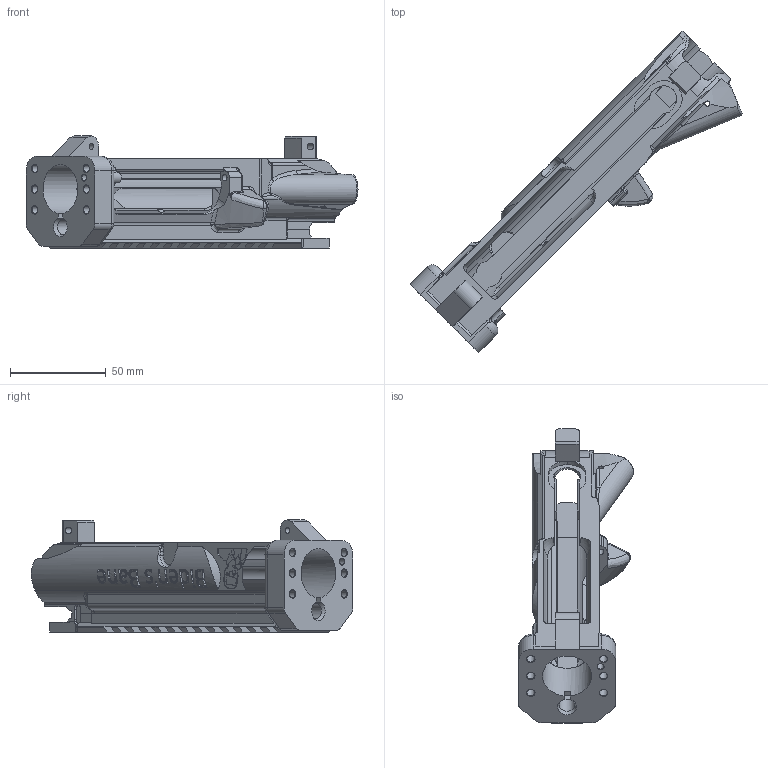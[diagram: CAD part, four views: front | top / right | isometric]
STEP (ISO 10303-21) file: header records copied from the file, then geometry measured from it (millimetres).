
FILE_DESCRIPTION(/* description */ ('STEP AP242','CAx-IF Rec.Pracs.---Representation and Presentation of Product Manufacturing Information (PMI)---4.0---2014-10-13','CAx-IF Rec.Pracs.---3D Tessellated Geometry---0.4---2014-09-14','2;1'),/* implementation_level */ '2;1');
FILE_NAME(/* name */ '62809140d1112b57fbcd074f',/* time_stamp */ '2022-05-15T05:36:02+00:00',/* author */ (''),/* organization */ (''),/* preprocessor_version */ 'ST-DEVELOPER v18.101',/* originating_system */ ' ',/* authorisation */ ' ');
FILE_SCHEMA (('AP242_MANAGED_MODEL_BASED_3D_ENGINEERING_MIM_LF { 1 0 10303 442 1 1 4 }'));
Length unit declared in the file: metre
Products named in the file (1): Imported1
Bounding box: 173.51 x 168.03 x 58.57 mm (x, y, z)
Volume: 121000.7 mm3; surface area: 56659.1 mm2
Topology: 1 solids, 2 shells, 1283 faces, 3588 edges, 2307 vertices
Faces by surface type: plane 733, bspline 321, cylinder 179, torus 22, cone 16, sphere 12
Full cylindrical faces by diameter (mm): 2.7 x1, 3.15 x1, 3.175 x1, 3.429 x2, 4.064 x6, 8 x1, 8.102 x1, 12.802 x1, 25.578 x1
Entity records: 44698 total; most frequent: CARTESIAN_POINT 14104, ORIENTED_EDGE 7056, DIRECTION 5145, EDGE_CURVE 3528, LINE 2355, VECTOR 2355, VERTEX_POINT 2295, AXIS2_PLACEMENT_3D 1395
